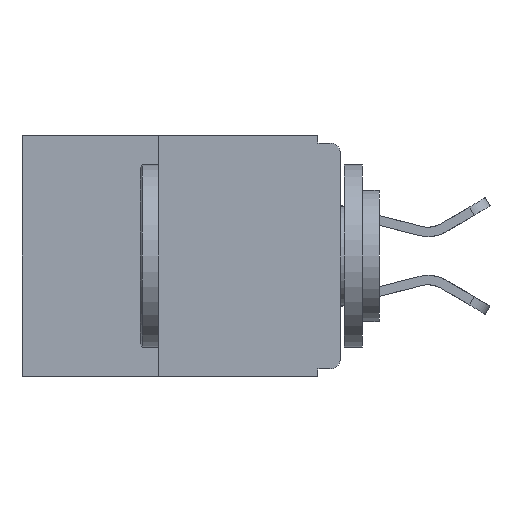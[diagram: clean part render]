
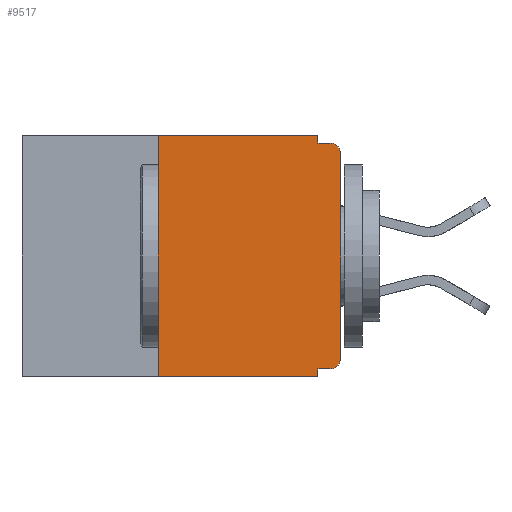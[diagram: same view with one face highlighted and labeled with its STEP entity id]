
A CAD part, left-side view. The second image highlights one B-rep face of the part: STEP entity #9517.
In plain terms, the highlighted planar face has unit normal (-1, 0, 0).
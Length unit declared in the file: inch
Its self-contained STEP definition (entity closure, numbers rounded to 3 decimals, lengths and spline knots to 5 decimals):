
#293 = LINE ( 'NONE', #3983, #6125 ) ;
#533 = EDGE_CURVE ( 'NONE', #13352, #13710, #8702, .T. ) ;
#783 = DIRECTION ( 'NONE',  ( 0., 0., -1. ) ) ;
#835 = CARTESIAN_POINT ( 'NONE',  ( 0., 0.031, 0. ) ) ;
#1409 = CARTESIAN_POINT ( 'NONE',  ( 0., 0.031, -0.01 ) ) ;
#1481 = DIRECTION ( 'NONE',  ( 0., -1., 0. ) ) ;
#1529 = CARTESIAN_POINT ( 'NONE',  ( 0., 0.25, -0.33 ) ) ;
#1684 = DIRECTION ( 'NONE',  ( 0., 0., 1. ) ) ;
#2523 = VERTEX_POINT ( 'NONE', #26967 ) ;
#2762 = ORIENTED_EDGE ( 'NONE', *, *, #5388, .F. ) ;
#2839 = VECTOR ( 'NONE', #12653, 39.37008 ) ;
#3314 = EDGE_LOOP ( 'NONE', ( #12117, #13704, #7822, #2762, #12697, #15277, #17952, #7989, #9823, #23660 ) ) ;
#3410 = CARTESIAN_POINT ( 'NONE',  ( 0., 0.015, -0.01 ) ) ;
#3418 = AXIS2_PLACEMENT_3D ( 'NONE', #4091, #4073, #4065 ) ;
#3748 = DIRECTION ( 'NONE',  ( -1., 0., 0. ) ) ;
#3983 = CARTESIAN_POINT ( 'NONE',  ( 0., 0.437, 0. ) ) ;
#4065 = DIRECTION ( 'NONE',  ( 0., 0., -1. ) ) ;
#4073 = DIRECTION ( 'NONE',  ( -1., 0., 0. ) ) ;
#4091 = CARTESIAN_POINT ( 'NONE',  ( 0., 0.015, -0.025 ) ) ;
#4371 = DIRECTION ( 'NONE',  ( 0., -1., 0. ) ) ;
#4858 = VECTOR ( 'NONE', #21040, 39.37008 ) ;
#5338 = VERTEX_POINT ( 'NONE', #1409 ) ;
#5388 = EDGE_CURVE ( 'NONE', #15463, #5338, #5636, .T. ) ;
#5603 = VERTEX_POINT ( 'NONE', #22863 ) ;
#5636 = LINE ( 'NONE', #835, #16997 ) ;
#5696 = CARTESIAN_POINT ( 'NONE',  ( 0., 0.25, -0.33 ) ) ;
#6092 = CARTESIAN_POINT ( 'NONE',  ( 0., 0., 0. ) ) ;
#6125 = VECTOR ( 'NONE', #4371, 39.37008 ) ;
#6464 = EDGE_CURVE ( 'NONE', #12076, #2523, #18637, .T. ) ;
#6612 = DIRECTION ( 'NONE',  ( 0., 0., 1. ) ) ;
#7196 = EDGE_CURVE ( 'NONE', #13710, #5603, #27378, .T. ) ;
#7621 = VECTOR ( 'NONE', #1684, 39.37008 ) ;
#7822 = ORIENTED_EDGE ( 'NONE', *, *, #21834, .F. ) ;
#7989 = ORIENTED_EDGE ( 'NONE', *, *, #7196, .F. ) ;
#8702 = LINE ( 'NONE', #17533, #2839 ) ;
#9517 = ADVANCED_FACE ( 'NONE', ( #10207 ), #23176, .F. ) ;
#9823 = ORIENTED_EDGE ( 'NONE', *, *, #533, .F. ) ;
#10094 = LINE ( 'NONE', #16454, #20691 ) ;
#10207 = FACE_OUTER_BOUND ( 'NONE', #3314, .T. ) ;
#11124 = VERTEX_POINT ( 'NONE', #3410 ) ;
#12076 = VERTEX_POINT ( 'NONE', #1529 ) ;
#12117 = ORIENTED_EDGE ( 'NONE', *, *, #18177, .T. ) ;
#12291 = CARTESIAN_POINT ( 'NONE',  ( 0., 0.437, -0.33 ) ) ;
#12653 = DIRECTION ( 'NONE',  ( 0., 1., 0. ) ) ;
#12697 = ORIENTED_EDGE ( 'NONE', *, *, #14617, .F. ) ;
#13252 = LINE ( 'NONE', #6092, #7621 ) ;
#13352 = VERTEX_POINT ( 'NONE', #22118 ) ;
#13704 = ORIENTED_EDGE ( 'NONE', *, *, #14607, .T. ) ;
#13710 = VERTEX_POINT ( 'NONE', #17149 ) ;
#13712 = LINE ( 'NONE', #12291, #24338 ) ;
#14607 = EDGE_CURVE ( 'NONE', #21733, #11124, #17488, .T. ) ;
#14617 = EDGE_CURVE ( 'NONE', #2523, #15463, #293, .T. ) ;
#15277 = ORIENTED_EDGE ( 'NONE', *, *, #6464, .F. ) ;
#15463 = VERTEX_POINT ( 'NONE', #23612 ) ;
#16454 = CARTESIAN_POINT ( 'NONE',  ( 0., 0., -0.01 ) ) ;
#16582 = CARTESIAN_POINT ( 'NONE',  ( 0., 0.015, -0.305 ) ) ;
#16997 = VECTOR ( 'NONE', #783, 39.37008 ) ;
#17149 = CARTESIAN_POINT ( 'NONE',  ( 0., 0.031, -0.32 ) ) ;
#17488 = CIRCLE ( 'NONE', #3418, 0.015 ) ;
#17533 = CARTESIAN_POINT ( 'NONE',  ( 0., 0., -0.32 ) ) ;
#17952 = ORIENTED_EDGE ( 'NONE', *, *, #25495, .T. ) ;
#17958 = VECTOR ( 'NONE', #6612, 39.37008 ) ;
#18047 = CARTESIAN_POINT ( 'NONE',  ( 0., 0., -0.305 ) ) ;
#18049 = CIRCLE ( 'NONE', #27417, 0.015 ) ;
#18177 = EDGE_CURVE ( 'NONE', #21035, #21733, #13252, .T. ) ;
#18286 = CARTESIAN_POINT ( 'NONE',  ( 0., 0., -0.025 ) ) ;
#18637 = LINE ( 'NONE', #5696, #17958 ) ;
#18783 = DIRECTION ( 'NONE',  ( 0., 0., -1. ) ) ;
#20691 = VECTOR ( 'NONE', #22873, 39.37008 ) ;
#21035 = VERTEX_POINT ( 'NONE', #18047 ) ;
#21040 = DIRECTION ( 'NONE',  ( 0., 0., -1. ) ) ;
#21254 = CARTESIAN_POINT ( 'NONE',  ( 0., 0.031, -0.33 ) ) ;
#21733 = VERTEX_POINT ( 'NONE', #18286 ) ;
#21834 = EDGE_CURVE ( 'NONE', #5338, #11124, #10094, .T. ) ;
#22118 = CARTESIAN_POINT ( 'NONE',  ( 0., 0.015, -0.32 ) ) ;
#22848 = DIRECTION ( 'NONE',  ( 0., 0., -1. ) ) ;
#22863 = CARTESIAN_POINT ( 'NONE',  ( 0., 0.031, -0.33 ) ) ;
#22873 = DIRECTION ( 'NONE',  ( 0., -1., 0. ) ) ;
#22878 = DIRECTION ( 'NONE',  ( 1., 0., 0. ) ) ;
#22979 = CARTESIAN_POINT ( 'NONE',  ( 0., 0.437, 0. ) ) ;
#23176 = PLANE ( 'NONE',  #25991 ) ;
#23612 = CARTESIAN_POINT ( 'NONE',  ( 0., 0.031, 0. ) ) ;
#23660 = ORIENTED_EDGE ( 'NONE', *, *, #26655, .T. ) ;
#24338 = VECTOR ( 'NONE', #1481, 39.37008 ) ;
#25495 = EDGE_CURVE ( 'NONE', #12076, #5603, #13712, .T. ) ;
#25991 = AXIS2_PLACEMENT_3D ( 'NONE', #22979, #22878, #22848 ) ;
#26655 = EDGE_CURVE ( 'NONE', #13352, #21035, #18049, .T. ) ;
#26967 = CARTESIAN_POINT ( 'NONE',  ( 0., 0.25, 0. ) ) ;
#27378 = LINE ( 'NONE', #21254, #4858 ) ;
#27417 = AXIS2_PLACEMENT_3D ( 'NONE', #16582, #3748, #18783 ) ;
